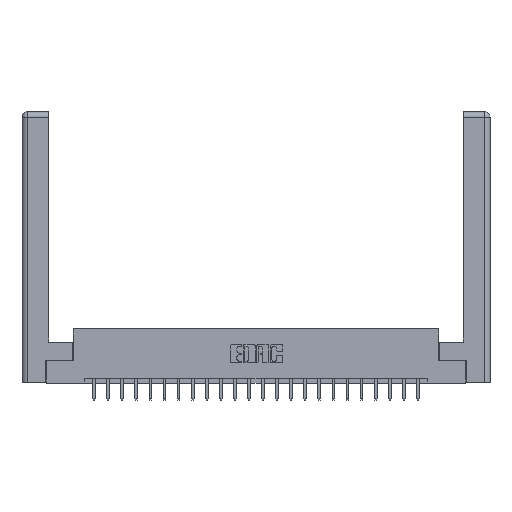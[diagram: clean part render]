
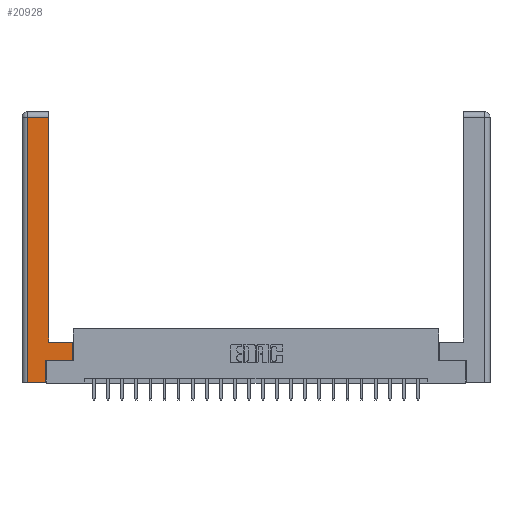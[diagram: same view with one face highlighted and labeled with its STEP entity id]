
A CAD part, top view. The second image highlights one B-rep face of the part: STEP entity #20928.
In plain terms, the highlighted planar face has unit normal (0, 0, 1).
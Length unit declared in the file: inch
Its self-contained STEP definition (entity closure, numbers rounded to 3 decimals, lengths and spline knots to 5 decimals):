
#75 = EDGE_CURVE ( 'NONE', #15540, #18028, #23706, .T. ) ;
#233 = VECTOR ( 'NONE', #7613, 39.37008 ) ;
#379 = EDGE_CURVE ( 'NONE', #11768, #8199, #16824, .T. ) ;
#1240 = LINE ( 'NONE', #4125, #10982 ) ;
#1338 = ORIENTED_EDGE ( 'NONE', *, *, #75, .T. ) ;
#1755 = DIRECTION ( 'NONE',  ( -1., 0., 0. ) ) ;
#2024 = VERTEX_POINT ( 'NONE', #22172 ) ;
#2626 = VERTEX_POINT ( 'NONE', #9003 ) ;
#3361 = LINE ( 'NONE', #13939, #22251 ) ;
#3528 = VECTOR ( 'NONE', #15264, 39.37008 ) ;
#3926 = VERTEX_POINT ( 'NONE', #21626 ) ;
#4125 = CARTESIAN_POINT ( 'NONE',  ( 0.265, 0., 0. ) ) ;
#4514 = ORIENTED_EDGE ( 'NONE', *, *, #19572, .T. ) ;
#4663 = CARTESIAN_POINT ( 'NONE',  ( 0.295, 2.94, 0. ) ) ;
#4675 = EDGE_CURVE ( 'NONE', #6309, #3926, #5547, .T. ) ;
#4939 = DIRECTION ( 'NONE',  ( 0., 1., 0. ) ) ;
#5281 = AXIS2_PLACEMENT_3D ( 'NONE', #19566, #12457, #8612 ) ;
#5547 = LINE ( 'NONE', #16163, #8443 ) ;
#5903 = CARTESIAN_POINT ( 'NONE',  ( 0.265, 0.245, 0. ) ) ;
#6309 = VERTEX_POINT ( 'NONE', #4663 ) ;
#6454 = DIRECTION ( 'NONE',  ( 1., 0., 0. ) ) ;
#6762 = PLANE ( 'NONE',  #5281 ) ;
#7469 = CARTESIAN_POINT ( 'NONE',  ( 0.565, 0.245, 0. ) ) ;
#7613 = DIRECTION ( 'NONE',  ( 0., -1., 0. ) ) ;
#7889 = DIRECTION ( 'NONE',  ( 1., 0., 0. ) ) ;
#7890 = FACE_OUTER_BOUND ( 'NONE', #21450, .T. ) ;
#8199 = VERTEX_POINT ( 'NONE', #17022 ) ;
#8443 = VECTOR ( 'NONE', #13944, 39.37008 ) ;
#8612 = DIRECTION ( 'NONE',  ( -1., 0., 0. ) ) ;
#9003 = CARTESIAN_POINT ( 'NONE',  ( 0.0615, 0., 0. ) ) ;
#9651 = ORIENTED_EDGE ( 'NONE', *, *, #14383, .T. ) ;
#10611 = ORIENTED_EDGE ( 'NONE', *, *, #13646, .T. ) ;
#10613 = ORIENTED_EDGE ( 'NONE', *, *, #15991, .T. ) ;
#10982 = VECTOR ( 'NONE', #7889, 39.37008 ) ;
#11118 = CARTESIAN_POINT ( 'NONE',  ( 0.295, 0.45, 0. ) ) ;
#11258 = LINE ( 'NONE', #21272, #21288 ) ;
#11768 = VERTEX_POINT ( 'NONE', #12899 ) ;
#12457 = DIRECTION ( 'NONE',  ( 0., 0., -1. ) ) ;
#12474 = ORIENTED_EDGE ( 'NONE', *, *, #4675, .T. ) ;
#12899 = CARTESIAN_POINT ( 'NONE',  ( 0.565, 0.45, 0. ) ) ;
#13436 = CARTESIAN_POINT ( 'NONE',  ( 0.265, 0.245, 0. ) ) ;
#13646 = EDGE_CURVE ( 'NONE', #2626, #2024, #1240, .T. ) ;
#13685 = ORIENTED_EDGE ( 'NONE', *, *, #19907, .T. ) ;
#13939 = CARTESIAN_POINT ( 'NONE',  ( 0.565, 0.45, 0. ) ) ;
#13944 = DIRECTION ( 'NONE',  ( -1., 0., 0. ) ) ;
#14217 = DIRECTION ( 'NONE',  ( 0., 1., 0. ) ) ;
#14383 = EDGE_CURVE ( 'NONE', #8199, #6309, #11258, .T. ) ;
#14576 = ORIENTED_EDGE ( 'NONE', *, *, #379, .T. ) ;
#14845 = LINE ( 'NONE', #20347, #233 ) ;
#15264 = DIRECTION ( 'NONE',  ( 0., 1., 0. ) ) ;
#15424 = VECTOR ( 'NONE', #6454, 39.37008 ) ;
#15540 = VERTEX_POINT ( 'NONE', #5903 ) ;
#15541 = LINE ( 'NONE', #13436, #3528 ) ;
#15991 = EDGE_CURVE ( 'NONE', #2024, #15540, #15541, .T. ) ;
#16163 = CARTESIAN_POINT ( 'NONE',  ( 0.0615, 2.94, 0. ) ) ;
#16824 = LINE ( 'NONE', #11118, #21124 ) ;
#17022 = CARTESIAN_POINT ( 'NONE',  ( 0.295, 0.45, 0. ) ) ;
#18028 = VERTEX_POINT ( 'NONE', #7469 ) ;
#19211 = CARTESIAN_POINT ( 'NONE',  ( 0.565, 0.245, 0. ) ) ;
#19566 = CARTESIAN_POINT ( 'NONE',  ( 0., 0., 0. ) ) ;
#19572 = EDGE_CURVE ( 'NONE', #3926, #2626, #14845, .T. ) ;
#19907 = EDGE_CURVE ( 'NONE', #18028, #11768, #3361, .T. ) ;
#20347 = CARTESIAN_POINT ( 'NONE',  ( 0.0615, 0., 0. ) ) ;
#20928 = ADVANCED_FACE ( 'NONE', ( #7890 ), #6762, .F. ) ;
#21124 = VECTOR ( 'NONE', #1755, 39.37008 ) ;
#21272 = CARTESIAN_POINT ( 'NONE',  ( 0.295, 3., 0. ) ) ;
#21288 = VECTOR ( 'NONE', #14217, 39.37008 ) ;
#21450 = EDGE_LOOP ( 'NONE', ( #9651, #12474, #4514, #10611, #10613, #1338, #13685, #14576 ) ) ;
#21626 = CARTESIAN_POINT ( 'NONE',  ( 0.0615, 2.94, 0. ) ) ;
#22172 = CARTESIAN_POINT ( 'NONE',  ( 0.265, 0., 0. ) ) ;
#22251 = VECTOR ( 'NONE', #4939, 39.37008 ) ;
#23706 = LINE ( 'NONE', #19211, #15424 ) ;
